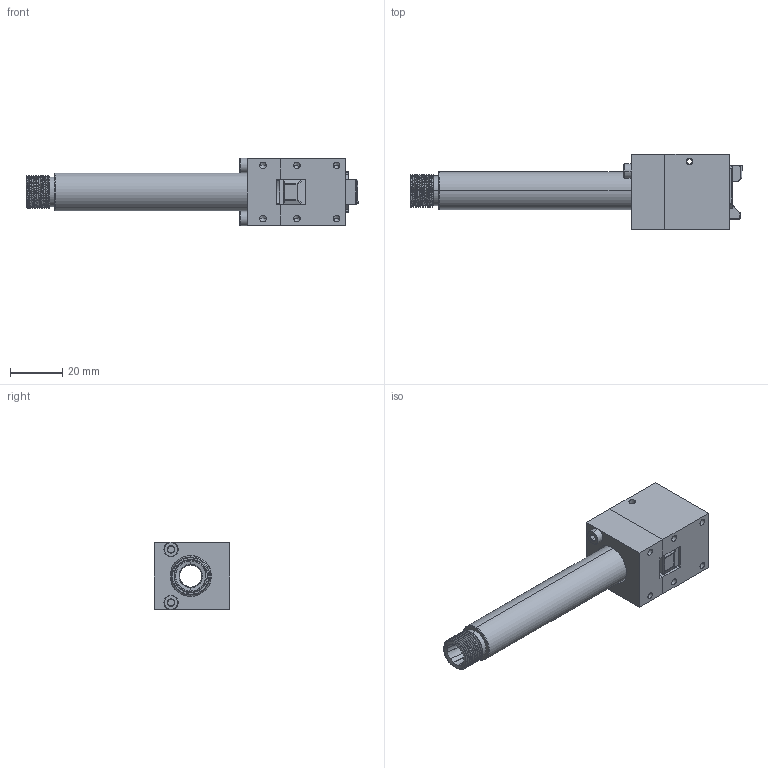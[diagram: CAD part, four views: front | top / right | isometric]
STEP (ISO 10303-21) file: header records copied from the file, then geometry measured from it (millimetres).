
FILE_DESCRIPTION (( 'STEP AP214' ), '1' );
FILE_NAME ('PPDW9 V4 Glock 17 Barrel and block.STEP', '2020-12-31T17:56:08', ( '' ), ( '' ), 'SwSTEP 2.0', 'SolidWorks 2020', '' );
FILE_SCHEMA (( 'AUTOMOTIVE_DESIGN' ));
Length unit declared in the file: inch
Products named in the file (5): Barrel Glock_17_Gen_1-4; PPDW9 V4 G17 barrel block; PPDW9 V4 Glock 17 Barrel and block; M3 x 25mm SHCS 91290A125_BLACK_91290A125; PPDW9 V4 G17 barrel block clamp
Assembly tree (5 placements, depth 2):
  PPDW9 V4 Glock 17 Barrel and block
    PPDW9 V4 G17 barrel block
    PPDW9 V4 G17 barrel block clamp
    Barrel Glock_17_Gen_1-4
    M3 x 25mm SHCS 91290A125_BLACK_91290A125  x2
Bounding box: 127 x 28.7 x 25.82 mm (x, y, z)
Volume: 31814 mm3; surface area: 21220.8 mm2
Topology: 5 solids, 5 shells, 1042 faces, 2845 edges, 1762 vertices
Faces by surface type: cylinder 516, bspline 261, plane 187, cone 67, torus 11
Entity records: 51376 total; most frequent: CARTESIAN_POINT 26330, ORIENTED_EDGE 4542, DIRECTION 2807, EDGE_CURVE 2271, VERTEX_POINT 1436, AXIS2_PLACEMENT_3D 979, EDGE_LOOP 899, FACE_OUTER_BOUND 865
